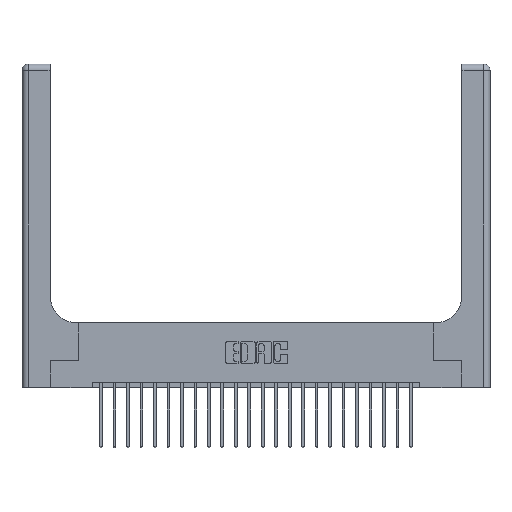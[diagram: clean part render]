
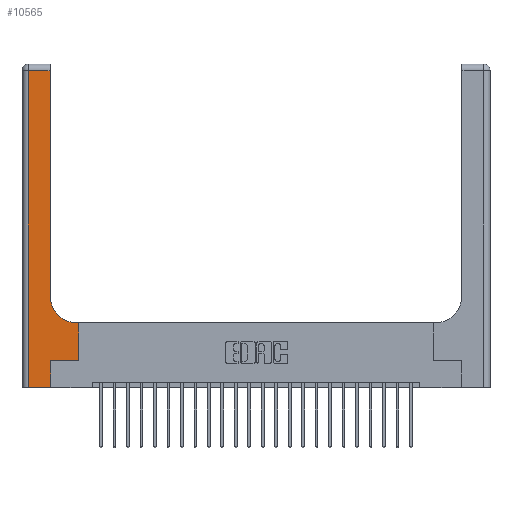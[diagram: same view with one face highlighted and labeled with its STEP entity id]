
A CAD part, top view. The second image highlights one B-rep face of the part: STEP entity #10565.
In plain terms, the highlighted planar face has unit normal (0, 0, 1).
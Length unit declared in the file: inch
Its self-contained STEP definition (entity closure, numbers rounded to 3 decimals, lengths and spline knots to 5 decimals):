
#82 = EDGE_CURVE ( 'NONE', #4482, #3422, #22097, .T. ) ;
#314 = VECTOR ( 'NONE', #10518, 39.37008 ) ;
#374 = CARTESIAN_POINT ( 'NONE',  ( 0.26, 0.85, 0.37 ) ) ;
#1057 = EDGE_CURVE ( 'NONE', #7684, #5665, #14482, .T. ) ;
#2709 = FACE_OUTER_BOUND ( 'NONE', #18227, .T. ) ;
#2814 = VECTOR ( 'NONE', #15873, 39.37008 ) ;
#2825 = DIRECTION ( 'NONE',  ( -1., 0., 0. ) ) ;
#2922 = VECTOR ( 'NONE', #4834, 39.37008 ) ;
#3422 = VERTEX_POINT ( 'NONE', #374 ) ;
#3717 = CARTESIAN_POINT ( 'NONE',  ( 0.26, 0.6, 0.37 ) ) ;
#3846 = EDGE_CURVE ( 'NONE', #11077, #4482, #5867, .T. ) ;
#4173 = EDGE_CURVE ( 'NONE', #14476, #9844, #12210, .T. ) ;
#4410 = EDGE_CURVE ( 'NONE', #9844, #10832, #6396, .T. ) ;
#4482 = VERTEX_POINT ( 'NONE', #6636 ) ;
#4834 = DIRECTION ( 'NONE',  ( 0., -1., 0. ) ) ;
#4892 = CARTESIAN_POINT ( 'NONE',  ( 0., 0., 0.37 ) ) ;
#5080 = LINE ( 'NONE', #23211, #2922 ) ;
#5239 = VECTOR ( 'NONE', #5380, 39.37008 ) ;
#5380 = DIRECTION ( 'NONE',  ( 1., 0., 0. ) ) ;
#5507 = ORIENTED_EDGE ( 'NONE', *, *, #4410, .T. ) ;
#5612 = CARTESIAN_POINT ( 'NONE',  ( 0.06, 2.94, 0.37 ) ) ;
#5665 = VERTEX_POINT ( 'NONE', #5612 ) ;
#5867 = LINE ( 'NONE', #3717, #15216 ) ;
#6294 = ORIENTED_EDGE ( 'NONE', *, *, #11874, .T. ) ;
#6299 = PLANE ( 'NONE',  #6687 ) ;
#6396 = LINE ( 'NONE', #10115, #2814 ) ;
#6400 = CARTESIAN_POINT ( 'NONE',  ( 0.06, 0., 0.37 ) ) ;
#6636 = CARTESIAN_POINT ( 'NONE',  ( 0.51, 0.6, 0.37 ) ) ;
#6687 = AXIS2_PLACEMENT_3D ( 'NONE', #13872, #17577, #2825 ) ;
#6746 = VECTOR ( 'NONE', #13021, 39.37008 ) ;
#7232 = CARTESIAN_POINT ( 'NONE',  ( 0.528, 0.6, 0.37 ) ) ;
#7293 = DIRECTION ( 'NONE',  ( 0., 1., 0. ) ) ;
#7476 = ORIENTED_EDGE ( 'NONE', *, *, #22759, .T. ) ;
#7635 = CARTESIAN_POINT ( 'NONE',  ( 0.265, 0., 0.37 ) ) ;
#7684 = VERTEX_POINT ( 'NONE', #12926 ) ;
#8859 = LINE ( 'NONE', #16175, #10179 ) ;
#8907 = CARTESIAN_POINT ( 'NONE',  ( 0.51, 0.85, 0.37 ) ) ;
#8916 = CARTESIAN_POINT ( 'NONE',  ( 0.528, 0.25, 0.37 ) ) ;
#9844 = VERTEX_POINT ( 'NONE', #7635 ) ;
#10115 = CARTESIAN_POINT ( 'NONE',  ( 0.265, 0., 0.37 ) ) ;
#10179 = VECTOR ( 'NONE', #7293, 39.37008 ) ;
#10518 = DIRECTION ( 'NONE',  ( -1., 0., 0. ) ) ;
#10565 = ADVANCED_FACE ( 'NONE', ( #2709 ), #6299, .F. ) ;
#10698 = DIRECTION ( 'NONE',  ( 1., 0., 0. ) ) ;
#10723 = ORIENTED_EDGE ( 'NONE', *, *, #3846, .T. ) ;
#10832 = VERTEX_POINT ( 'NONE', #15042 ) ;
#11055 = ORIENTED_EDGE ( 'NONE', *, *, #23061, .T. ) ;
#11077 = VERTEX_POINT ( 'NONE', #7232 ) ;
#11161 = ORIENTED_EDGE ( 'NONE', *, *, #4173, .T. ) ;
#11717 = AXIS2_PLACEMENT_3D ( 'NONE', #8907, #23669, #10698 ) ;
#11874 = EDGE_CURVE ( 'NONE', #12229, #11077, #8859, .T. ) ;
#12210 = LINE ( 'NONE', #4892, #5239 ) ;
#12229 = VERTEX_POINT ( 'NONE', #8916 ) ;
#12926 = CARTESIAN_POINT ( 'NONE',  ( 0.26, 2.94, 0.37 ) ) ;
#12969 = EDGE_CURVE ( 'NONE', #10832, #12229, #17143, .T. ) ;
#13021 = DIRECTION ( 'NONE',  ( 0., 1., 0. ) ) ;
#13360 = ORIENTED_EDGE ( 'NONE', *, *, #1057, .T. ) ;
#13872 = CARTESIAN_POINT ( 'NONE',  ( 0., 3., 0.37 ) ) ;
#14223 = ORIENTED_EDGE ( 'NONE', *, *, #12969, .T. ) ;
#14455 = LINE ( 'NONE', #16612, #6746 ) ;
#14476 = VERTEX_POINT ( 'NONE', #6400 ) ;
#14482 = LINE ( 'NONE', #15929, #314 ) ;
#15042 = CARTESIAN_POINT ( 'NONE',  ( 0.265, 0.25, 0.37 ) ) ;
#15216 = VECTOR ( 'NONE', #22086, 39.37008 ) ;
#15873 = DIRECTION ( 'NONE',  ( 0., 1., 0. ) ) ;
#15929 = CARTESIAN_POINT ( 'NONE',  ( 0., 2.94, 0.37 ) ) ;
#15982 = VECTOR ( 'NONE', #19297, 39.37008 ) ;
#16175 = CARTESIAN_POINT ( 'NONE',  ( 0.528, 0.25, 0.37 ) ) ;
#16612 = CARTESIAN_POINT ( 'NONE',  ( 0.26, 3., 0.37 ) ) ;
#17143 = LINE ( 'NONE', #19058, #15982 ) ;
#17577 = DIRECTION ( 'NONE',  ( 0., 0., -1. ) ) ;
#18227 = EDGE_LOOP ( 'NONE', ( #7476, #13360, #11055, #11161, #5507, #14223, #6294, #10723, #21073 ) ) ;
#19058 = CARTESIAN_POINT ( 'NONE',  ( 0.265, 0.25, 0.37 ) ) ;
#19297 = DIRECTION ( 'NONE',  ( 1., 0., 0. ) ) ;
#21073 = ORIENTED_EDGE ( 'NONE', *, *, #82, .T. ) ;
#22086 = DIRECTION ( 'NONE',  ( -1., 0., 0. ) ) ;
#22097 = CIRCLE ( 'NONE', #11717, 0.25 ) ;
#22759 = EDGE_CURVE ( 'NONE', #3422, #7684, #14455, .T. ) ;
#23061 = EDGE_CURVE ( 'NONE', #5665, #14476, #5080, .T. ) ;
#23211 = CARTESIAN_POINT ( 'NONE',  ( 0.06, 3., 0.37 ) ) ;
#23669 = DIRECTION ( 'NONE',  ( 0., 0., -1. ) ) ;
